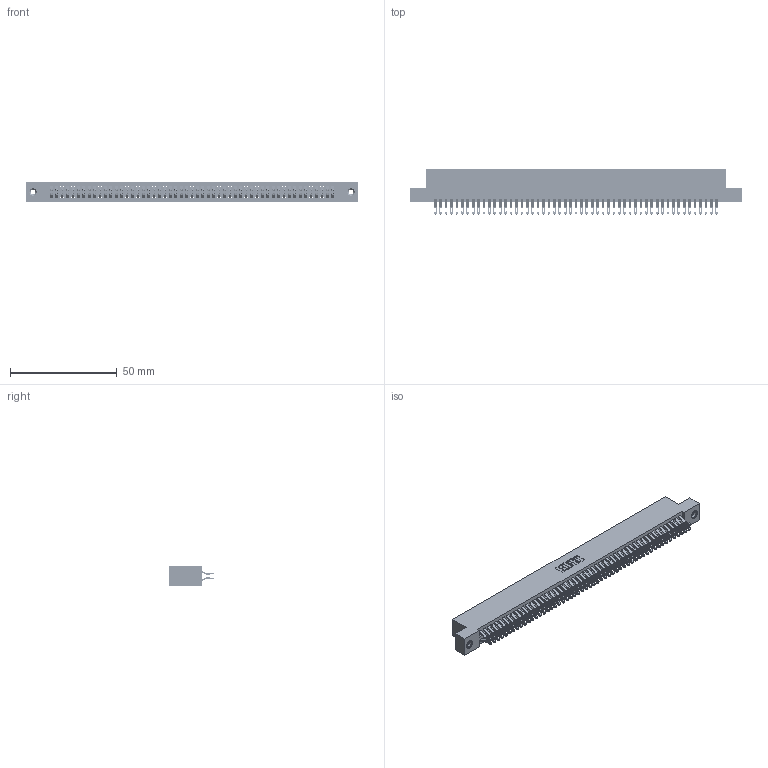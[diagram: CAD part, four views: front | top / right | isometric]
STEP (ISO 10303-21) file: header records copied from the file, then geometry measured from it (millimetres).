
FILE_DESCRIPTION (( 'STEP AP203' ), '1' );
FILE_NAME ('345-106-555-208.STEP', '2019-11-03T16:57:55', ( '' ), ( '' ), 'SwSTEP 2.0', 'SolidWorks 2016', '' );
FILE_SCHEMA (( 'CONFIG_CONTROL_DESIGN' ));
Length unit declared in the file: inch
Products named in the file (4): 345-106-555-208; 345-250-001_345-250-003-102; 345-292-001_555 Tail; 345 Part_Flush Mounting Lugs - 0.156 Dia-TI
Assembly tree (109 placements, depth 2):
  345-106-555-208
    345 Part_Flush Mounting Lugs - 0.156 Dia-TI
    345-292-001_555 Tail  x106
    345-250-001_345-250-003-102  x2
Bounding box: 155.83 x 21.13 x 9.4 mm (x, y, z)
Volume: 15540.4 mm3; surface area: 24267.2 mm2
Topology: 109 solids, 109 shells, 6122 faces, 19239 edges, 12818 vertices
Faces by surface type: plane 3398, cylinder 2708, cone 12, torus 4
Entity records: 41616 total; most frequent: CARTESIAN_POINT 6981, ORIENTED_EDGE 6878, DIRECTION 6137, EDGE_CURVE 3439, LINE 3055, VECTOR 3055, VERTEX_POINT 2288, AXIS2_PLACEMENT_3D 1541
